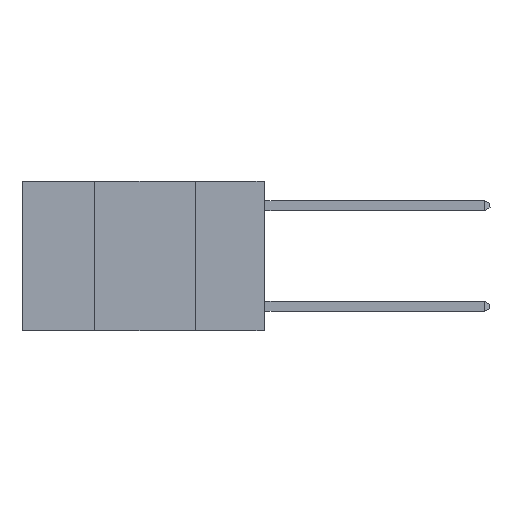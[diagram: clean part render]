
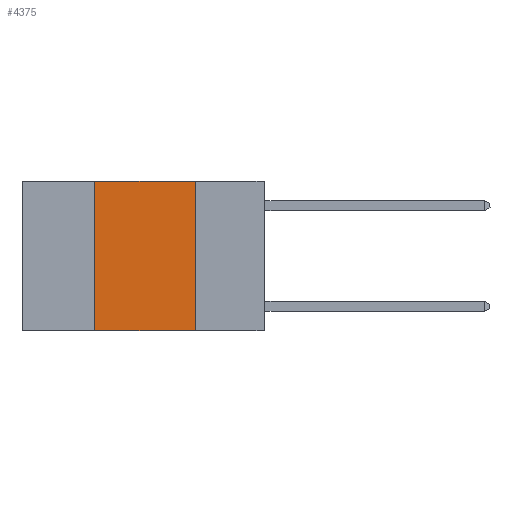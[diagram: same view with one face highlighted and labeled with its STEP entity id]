
A CAD part, left-side view. The second image highlights one B-rep face of the part: STEP entity #4375.
In plain terms, the highlighted planar face has unit normal (-1, 0, 0).
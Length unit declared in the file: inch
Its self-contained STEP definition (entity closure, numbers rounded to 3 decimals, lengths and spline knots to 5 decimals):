
#72 = VECTOR ( 'NONE', #8378, 39.37008 ) ;
#289 = DIRECTION ( 'NONE',  ( 0., 0., 1. ) ) ;
#359 = CARTESIAN_POINT ( 'NONE',  ( 0., 0.17, 0. ) ) ;
#926 = EDGE_LOOP ( 'NONE', ( #1779, #4902, #4456, #5835 ) ) ;
#1181 = LINE ( 'NONE', #1440, #8322 ) ;
#1440 = CARTESIAN_POINT ( 'NONE',  ( 0., 0.6, 0. ) ) ;
#1617 = VERTEX_POINT ( 'NONE', #4919 ) ;
#1779 = ORIENTED_EDGE ( 'NONE', *, *, #4195, .F. ) ;
#1940 = LINE ( 'NONE', #8565, #8799 ) ;
#2038 = CARTESIAN_POINT ( 'NONE',  ( 0., 0.17, 0. ) ) ;
#2280 = LINE ( 'NONE', #2038, #5853 ) ;
#2551 = VERTEX_POINT ( 'NONE', #8524 ) ;
#2735 = DIRECTION ( 'NONE',  ( 0., 0., -1. ) ) ;
#3810 = CARTESIAN_POINT ( 'NONE',  ( 0., 0.42, -0.37 ) ) ;
#3921 = DIRECTION ( 'NONE',  ( 0., 0., -1. ) ) ;
#3947 = VERTEX_POINT ( 'NONE', #3810 ) ;
#4195 = EDGE_CURVE ( 'NONE', #7230, #2551, #2280, .T. ) ;
#4375 = ADVANCED_FACE ( 'NONE', ( #7096 ), #6011, .F. ) ;
#4456 = ORIENTED_EDGE ( 'NONE', *, *, #4682, .F. ) ;
#4682 = EDGE_CURVE ( 'NONE', #3947, #1617, #1940, .T. ) ;
#4902 = ORIENTED_EDGE ( 'NONE', *, *, #6165, .F. ) ;
#4919 = CARTESIAN_POINT ( 'NONE',  ( 0., 0.42, 0. ) ) ;
#5326 = CARTESIAN_POINT ( 'NONE',  ( 0., 0.6, 0. ) ) ;
#5751 = LINE ( 'NONE', #7732, #72 ) ;
#5835 = ORIENTED_EDGE ( 'NONE', *, *, #7793, .T. ) ;
#5853 = VECTOR ( 'NONE', #2735, 39.37008 ) ;
#6011 = PLANE ( 'NONE',  #8076 ) ;
#6165 = EDGE_CURVE ( 'NONE', #1617, #7230, #1181, .T. ) ;
#7055 = DIRECTION ( 'NONE',  ( 0., -1., 0. ) ) ;
#7096 = FACE_OUTER_BOUND ( 'NONE', #926, .T. ) ;
#7230 = VERTEX_POINT ( 'NONE', #359 ) ;
#7732 = CARTESIAN_POINT ( 'NONE',  ( 0., 0.6, -0.37 ) ) ;
#7793 = EDGE_CURVE ( 'NONE', #3947, #2551, #5751, .T. ) ;
#7975 = DIRECTION ( 'NONE',  ( 1., 0., 0. ) ) ;
#8076 = AXIS2_PLACEMENT_3D ( 'NONE', #5326, #7975, #3921 ) ;
#8322 = VECTOR ( 'NONE', #7055, 39.37008 ) ;
#8378 = DIRECTION ( 'NONE',  ( 0., -1., 0. ) ) ;
#8524 = CARTESIAN_POINT ( 'NONE',  ( 0., 0.17, -0.37 ) ) ;
#8565 = CARTESIAN_POINT ( 'NONE',  ( 0., 0.42, 0. ) ) ;
#8799 = VECTOR ( 'NONE', #289, 39.37008 ) ;
